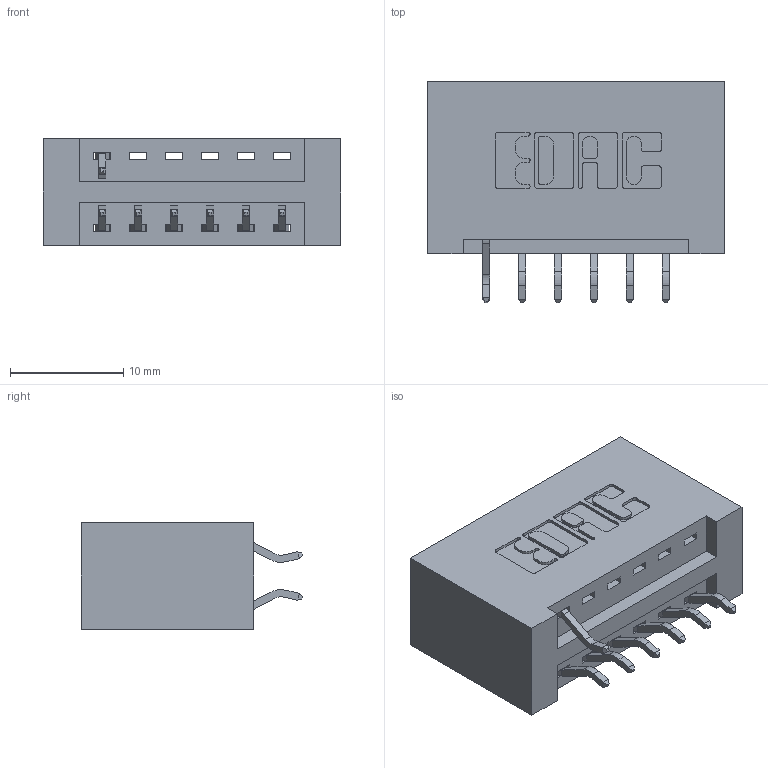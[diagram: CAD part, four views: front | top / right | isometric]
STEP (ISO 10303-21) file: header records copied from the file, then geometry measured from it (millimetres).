
FILE_DESCRIPTION (( 'STEP AP203' ), '1' );
FILE_NAME ('346-012-556-201.STEP', '2018-08-19T22:51:34', ( '' ), ( '' ), 'SwSTEP 2.0', 'SolidWorks 2016', '' );
FILE_SCHEMA (( 'CONFIG_CONTROL_DESIGN' ));
Length unit declared in the file: inch
Products named in the file (3): 346 Part_No Mounting Lugs; 345-292-001_556 Tail; 346-012-556-201
Assembly tree (8 placements, depth 2):
  346-012-556-201
    346 Part_No Mounting Lugs
    345-292-001_556 Tail  x7
Bounding box: 26.29 x 19.57 x 9.4 mm (x, y, z)
Volume: 2811.9 mm3; surface area: 3196.5 mm2
Topology: 8 solids, 8 shells, 550 faces, 1621 edges, 1070 vertices
Faces by surface type: plane 370, cylinder 180
Entity records: 8545 total; most frequent: CARTESIAN_POINT 1491, ORIENTED_EDGE 1418, DIRECTION 1343, EDGE_CURVE 709, VECTOR 553, LINE 553, VERTEX_POINT 470, AXIS2_PLACEMENT_3D 395
